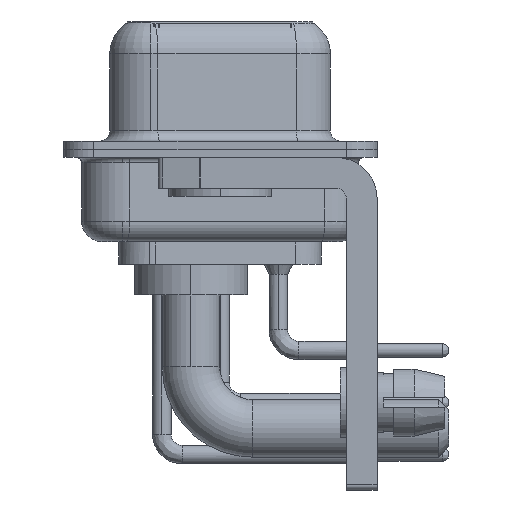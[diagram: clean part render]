
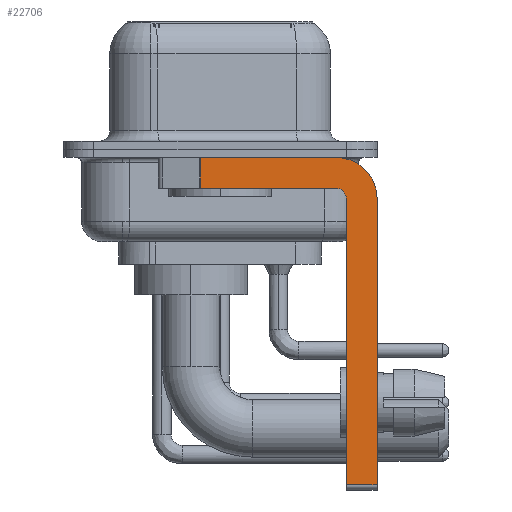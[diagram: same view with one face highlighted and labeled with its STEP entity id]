
A CAD part, left-side view. The second image highlights one B-rep face of the part: STEP entity #22706.
In plain terms, the highlighted planar face has unit normal (-1, 0, 0).
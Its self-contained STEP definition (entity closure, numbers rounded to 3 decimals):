
#400 = DIRECTION ( 'NONE',  ( 0., -1., 0. ) ) ;
#783 = VECTOR ( 'NONE', #19859, 1000. ) ;
#986 = LINE ( 'NONE', #22673, #7807 ) ;
#1047 = EDGE_CURVE ( 'NONE', #17456, #16636, #19519, .T. ) ;
#1111 = CARTESIAN_POINT ( 'NONE',  ( -2.9, -6.15, -16.35 ) ) ;
#1169 = CARTESIAN_POINT ( 'NONE',  ( -2.9, 3., -0.4 ) ) ;
#2937 = VECTOR ( 'NONE', #30304, 1000. ) ;
#3113 = CARTESIAN_POINT ( 'NONE',  ( -2.9, -6.15, -2.4 ) ) ;
#5658 = VECTOR ( 'NONE', #14375, 1000. ) ;
#7307 = EDGE_LOOP ( 'NONE', ( #17436, #30410, #20079, #18097, #30986, #33696, #33527, #13611 ) ) ;
#7320 = EDGE_CURVE ( 'NONE', #14311, #16636, #19670, .T. ) ;
#7807 = VECTOR ( 'NONE', #33107, 1000. ) ;
#8528 = CARTESIAN_POINT ( 'NONE',  ( -2.9, -7.65, -2.4 ) ) ;
#9134 = LINE ( 'NONE', #1169, #783 ) ;
#10038 = DIRECTION ( 'NONE',  ( 1., 0., 0. ) ) ;
#10391 = CARTESIAN_POINT ( 'NONE',  ( -2.9, -5.65, -2.4 ) ) ;
#10733 = DIRECTION ( 'NONE',  ( 0., 0., -1. ) ) ;
#10748 = VECTOR ( 'NONE', #400, 1000. ) ;
#11274 = CIRCLE ( 'NONE', #33794, 0.5 ) ;
#11328 = CARTESIAN_POINT ( 'NONE',  ( -2.9, -5.65, -1.9 ) ) ;
#13018 = FACE_OUTER_BOUND ( 'NONE', #7307, .T. ) ;
#13611 = ORIENTED_EDGE ( 'NONE', *, *, #18644, .F. ) ;
#13768 = DIRECTION ( 'NONE',  ( 0., 0., 1. ) ) ;
#14287 = CARTESIAN_POINT ( 'NONE',  ( -2.9, 0.978, -0.4 ) ) ;
#14311 = VERTEX_POINT ( 'NONE', #14287 ) ;
#14375 = DIRECTION ( 'NONE',  ( 0., 0., -1. ) ) ;
#14668 = VERTEX_POINT ( 'NONE', #29613 ) ;
#14739 = EDGE_CURVE ( 'NONE', #25219, #17456, #11274, .T. ) ;
#15454 = EDGE_CURVE ( 'NONE', #34001, #28964, #18573, .T. ) ;
#15643 = AXIS2_PLACEMENT_3D ( 'NONE', #18452, #18628, #26757 ) ;
#16062 = CARTESIAN_POINT ( 'NONE',  ( -2.9, -7.65, -16.35 ) ) ;
#16636 = VERTEX_POINT ( 'NONE', #30786 ) ;
#17436 = ORIENTED_EDGE ( 'NONE', *, *, #23111, .F. ) ;
#17456 = VERTEX_POINT ( 'NONE', #11328 ) ;
#18097 = ORIENTED_EDGE ( 'NONE', *, *, #14739, .F. ) ;
#18452 = CARTESIAN_POINT ( 'NONE',  ( -2.9, -5.65, -2.4 ) ) ;
#18573 = LINE ( 'NONE', #18748, #10748 ) ;
#18628 = DIRECTION ( 'NONE',  ( 1., 0., 0. ) ) ;
#18644 = EDGE_CURVE ( 'NONE', #14668, #25985, #24080, .T. ) ;
#18748 = CARTESIAN_POINT ( 'NONE',  ( -2.9, -5.65, -16.35 ) ) ;
#18916 = EDGE_CURVE ( 'NONE', #25985, #28964, #986, .T. ) ;
#19519 = LINE ( 'NONE', #25522, #2937 ) ;
#19570 = LINE ( 'NONE', #29833, #27378 ) ;
#19670 = LINE ( 'NONE', #30458, #5658 ) ;
#19859 = DIRECTION ( 'NONE',  ( 0., -1., 0. ) ) ;
#20079 = ORIENTED_EDGE ( 'NONE', *, *, #1047, .F. ) ;
#22150 = AXIS2_PLACEMENT_3D ( 'NONE', #10391, #10038, #10733 ) ;
#22673 = CARTESIAN_POINT ( 'NONE',  ( -2.9, -7.65, -2.4 ) ) ;
#22706 = ADVANCED_FACE ( 'NONE', ( #13018 ), #26250, .F. ) ;
#23111 = EDGE_CURVE ( 'NONE', #14311, #14668, #9134, .T. ) ;
#24080 = CIRCLE ( 'NONE', #15643, 2. ) ;
#25168 = DIRECTION ( 'NONE',  ( 0., 0., 1. ) ) ;
#25219 = VERTEX_POINT ( 'NONE', #3113 ) ;
#25522 = CARTESIAN_POINT ( 'NONE',  ( -2.9, -5.65, -1.9 ) ) ;
#25985 = VERTEX_POINT ( 'NONE', #8528 ) ;
#26250 = PLANE ( 'NONE',  #22150 ) ;
#26757 = DIRECTION ( 'NONE',  ( 0., 0., -1. ) ) ;
#27378 = VECTOR ( 'NONE', #13768, 1000. ) ;
#28964 = VERTEX_POINT ( 'NONE', #16062 ) ;
#29613 = CARTESIAN_POINT ( 'NONE',  ( -2.9, -5.65, -0.4 ) ) ;
#29833 = CARTESIAN_POINT ( 'NONE',  ( -2.9, -6.15, -16.6 ) ) ;
#30304 = DIRECTION ( 'NONE',  ( 0., 1., 0. ) ) ;
#30410 = ORIENTED_EDGE ( 'NONE', *, *, #7320, .T. ) ;
#30458 = CARTESIAN_POINT ( 'NONE',  ( -2.9, 0.978, -1.9 ) ) ;
#30786 = CARTESIAN_POINT ( 'NONE',  ( -2.9, 0.978, -1.9 ) ) ;
#30986 = ORIENTED_EDGE ( 'NONE', *, *, #32330, .F. ) ;
#32330 = EDGE_CURVE ( 'NONE', #34001, #25219, #19570, .T. ) ;
#32963 = CARTESIAN_POINT ( 'NONE',  ( -2.9, -5.65, -2.4 ) ) ;
#33107 = DIRECTION ( 'NONE',  ( 0., 0., -1. ) ) ;
#33139 = DIRECTION ( 'NONE',  ( -1., 0., 0. ) ) ;
#33527 = ORIENTED_EDGE ( 'NONE', *, *, #18916, .F. ) ;
#33696 = ORIENTED_EDGE ( 'NONE', *, *, #15454, .T. ) ;
#33794 = AXIS2_PLACEMENT_3D ( 'NONE', #32963, #33139, #25168 ) ;
#34001 = VERTEX_POINT ( 'NONE', #1111 ) ;
